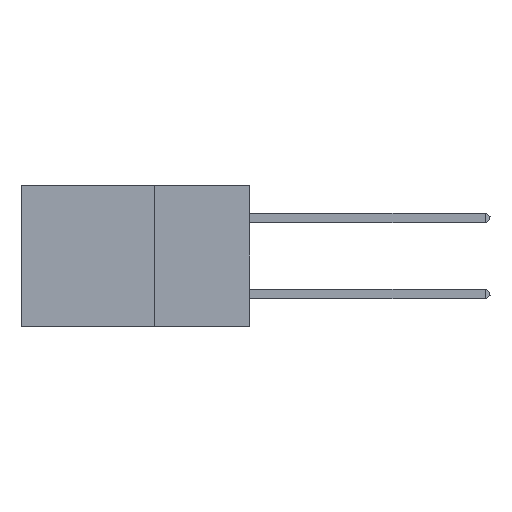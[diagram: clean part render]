
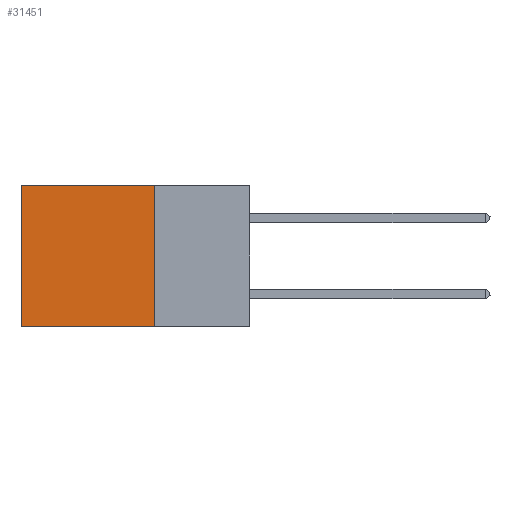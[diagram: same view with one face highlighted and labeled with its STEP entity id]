
A CAD part, left-side view. The second image highlights one B-rep face of the part: STEP entity #31451.
In plain terms, the highlighted planar face has unit normal (-1, 0, 0).
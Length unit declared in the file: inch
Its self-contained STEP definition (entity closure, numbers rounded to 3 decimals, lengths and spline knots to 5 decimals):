
#3601 = CARTESIAN_POINT ( 'NONE',  ( 0.2875, 0.25, 0. ) ) ;
#4244 = CARTESIAN_POINT ( 'NONE',  ( 0.2875, 0.6, 0. ) ) ;
#6821 = EDGE_CURVE ( 'NONE', #11530, #7863, #27952, .T. ) ;
#7863 = VERTEX_POINT ( 'NONE', #25956 ) ;
#8594 = DIRECTION ( 'NONE',  ( 0., 1., 0. ) ) ;
#8637 = EDGE_CURVE ( 'NONE', #16963, #30658, #20966, .T. ) ;
#9366 = DIRECTION ( 'NONE',  ( 0., 1., 0. ) ) ;
#10533 = ORIENTED_EDGE ( 'NONE', *, *, #29595, .T. ) ;
#11530 = VERTEX_POINT ( 'NONE', #18129 ) ;
#12527 = DIRECTION ( 'NONE',  ( 0., 0., -1. ) ) ;
#12717 = CARTESIAN_POINT ( 'NONE',  ( 0.2875, 0.25, 0. ) ) ;
#13089 = AXIS2_PLACEMENT_3D ( 'NONE', #3601, #25621, #20060 ) ;
#13647 = ORIENTED_EDGE ( 'NONE', *, *, #6821, .T. ) ;
#15125 = DIRECTION ( 'NONE',  ( 0., 0., -1. ) ) ;
#15393 = LINE ( 'NONE', #4244, #19222 ) ;
#15753 = LINE ( 'NONE', #12717, #24815 ) ;
#16963 = VERTEX_POINT ( 'NONE', #26975 ) ;
#17212 = EDGE_LOOP ( 'NONE', ( #10533, #24706, #24487, #13647 ) ) ;
#18129 = CARTESIAN_POINT ( 'NONE',  ( 0.2875, 0.25, 0. ) ) ;
#19222 = VECTOR ( 'NONE', #12527, 39.37008 ) ;
#20060 = DIRECTION ( 'NONE',  ( 0., 0., -1. ) ) ;
#20966 = LINE ( 'NONE', #27285, #29536 ) ;
#22750 = PLANE ( 'NONE',  #13089 ) ;
#23943 = FACE_OUTER_BOUND ( 'NONE', #17212, .T. ) ;
#24487 = ORIENTED_EDGE ( 'NONE', *, *, #30281, .F. ) ;
#24706 = ORIENTED_EDGE ( 'NONE', *, *, #8637, .F. ) ;
#24815 = VECTOR ( 'NONE', #15125, 39.37008 ) ;
#25371 = VECTOR ( 'NONE', #9366, 39.37008 ) ;
#25621 = DIRECTION ( 'NONE',  ( 1., 0., 0. ) ) ;
#25909 = CARTESIAN_POINT ( 'NONE',  ( 0.2875, 0.6, -0.37 ) ) ;
#25956 = CARTESIAN_POINT ( 'NONE',  ( 0.2875, 0.6, 0. ) ) ;
#26975 = CARTESIAN_POINT ( 'NONE',  ( 0.2875, 0.25, -0.37 ) ) ;
#27285 = CARTESIAN_POINT ( 'NONE',  ( 0.2875, 0.25, -0.37 ) ) ;
#27952 = LINE ( 'NONE', #30887, #25371 ) ;
#29536 = VECTOR ( 'NONE', #8594, 39.37008 ) ;
#29595 = EDGE_CURVE ( 'NONE', #7863, #30658, #15393, .T. ) ;
#30281 = EDGE_CURVE ( 'NONE', #11530, #16963, #15753, .T. ) ;
#30658 = VERTEX_POINT ( 'NONE', #25909 ) ;
#30887 = CARTESIAN_POINT ( 'NONE',  ( 0.2875, 0.25, 0. ) ) ;
#31451 = ADVANCED_FACE ( 'NONE', ( #23943 ), #22750, .F. ) ;
